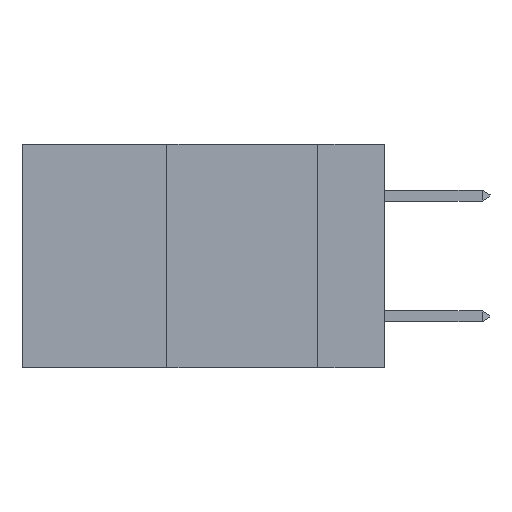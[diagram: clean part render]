
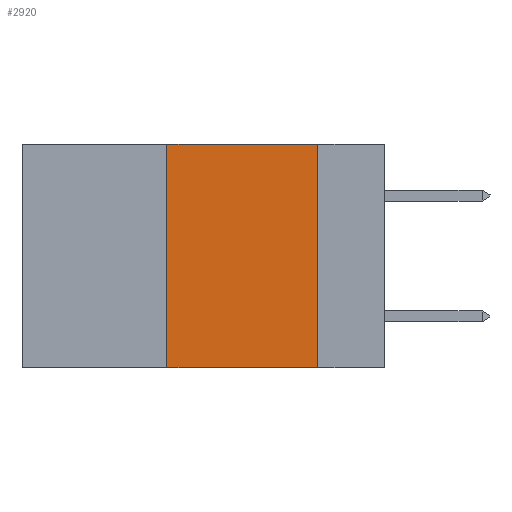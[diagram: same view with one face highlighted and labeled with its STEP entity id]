
A CAD part, left-side view. The second image highlights one B-rep face of the part: STEP entity #2920.
In plain terms, the highlighted planar face has unit normal (-1, 0, 0).
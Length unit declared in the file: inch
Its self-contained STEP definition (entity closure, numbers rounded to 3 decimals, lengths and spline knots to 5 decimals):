
#846 = FACE_OUTER_BOUND ( 'NONE', #8473, .T. ) ;
#1207 = CARTESIAN_POINT ( 'NONE',  ( 0., 0.36, 0. ) ) ;
#1700 = CARTESIAN_POINT ( 'NONE',  ( 0., 0.6, 0. ) ) ;
#2920 = ADVANCED_FACE ( 'NONE', ( #846 ), #33317, .F. ) ;
#3263 = ORIENTED_EDGE ( 'NONE', *, *, #22485, .T. ) ;
#3470 = CARTESIAN_POINT ( 'NONE',  ( 0., 0.6, -0.37 ) ) ;
#4738 = DIRECTION ( 'NONE',  ( 0., 0., -1. ) ) ;
#6236 = CARTESIAN_POINT ( 'NONE',  ( 0., 0.6, 0. ) ) ;
#6437 = ORIENTED_EDGE ( 'NONE', *, *, #43408, .F. ) ;
#8473 = EDGE_LOOP ( 'NONE', ( #6437, #19738, #26142, #3263 ) ) ;
#11087 = CARTESIAN_POINT ( 'NONE',  ( 0., 0.36, 0. ) ) ;
#18858 = VERTEX_POINT ( 'NONE', #1207 ) ;
#19018 = VERTEX_POINT ( 'NONE', #24440 ) ;
#19108 = EDGE_CURVE ( 'NONE', #19018, #18858, #30986, .T. ) ;
#19157 = DIRECTION ( 'NONE',  ( 1., 0., 0. ) ) ;
#19738 = ORIENTED_EDGE ( 'NONE', *, *, #29979, .F. ) ;
#19934 = LINE ( 'NONE', #24103, #31481 ) ;
#20584 = CARTESIAN_POINT ( 'NONE',  ( 0., 0.11, -0.37 ) ) ;
#21254 = VECTOR ( 'NONE', #42143, 39.37008 ) ;
#21500 = CARTESIAN_POINT ( 'NONE',  ( 0., 0.11, 0. ) ) ;
#22485 = EDGE_CURVE ( 'NONE', #19018, #41417, #25067, .T. ) ;
#24103 = CARTESIAN_POINT ( 'NONE',  ( 0., 0.11, 0. ) ) ;
#24440 = CARTESIAN_POINT ( 'NONE',  ( 0., 0.36, -0.37 ) ) ;
#25067 = LINE ( 'NONE', #3470, #21254 ) ;
#26142 = ORIENTED_EDGE ( 'NONE', *, *, #19108, .F. ) ;
#29979 = EDGE_CURVE ( 'NONE', #18858, #33307, #34406, .T. ) ;
#30986 = LINE ( 'NONE', #11087, #39236 ) ;
#31481 = VECTOR ( 'NONE', #34404, 39.37008 ) ;
#33307 = VERTEX_POINT ( 'NONE', #21500 ) ;
#33310 = VECTOR ( 'NONE', #44914, 39.37008 ) ;
#33317 = PLANE ( 'NONE',  #40028 ) ;
#34404 = DIRECTION ( 'NONE',  ( 0., 0., -1. ) ) ;
#34406 = LINE ( 'NONE', #6236, #33310 ) ;
#39236 = VECTOR ( 'NONE', #42826, 39.37008 ) ;
#40028 = AXIS2_PLACEMENT_3D ( 'NONE', #1700, #19157, #4738 ) ;
#41417 = VERTEX_POINT ( 'NONE', #20584 ) ;
#42143 = DIRECTION ( 'NONE',  ( 0., -1., 0. ) ) ;
#42826 = DIRECTION ( 'NONE',  ( 0., 0., 1. ) ) ;
#43408 = EDGE_CURVE ( 'NONE', #33307, #41417, #19934, .T. ) ;
#44914 = DIRECTION ( 'NONE',  ( 0., -1., 0. ) ) ;
